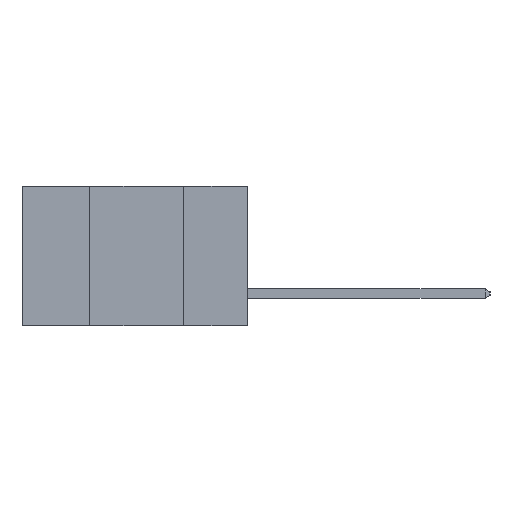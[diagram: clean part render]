
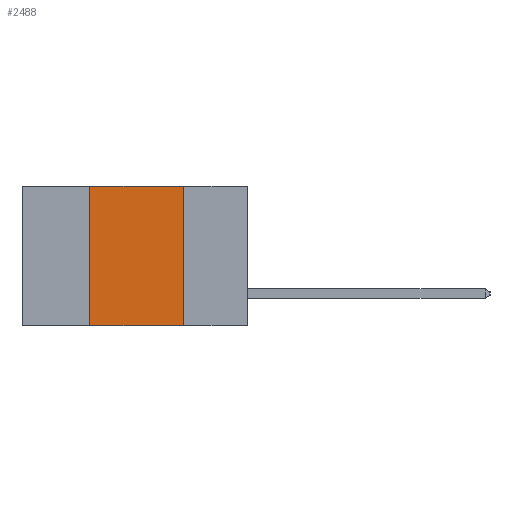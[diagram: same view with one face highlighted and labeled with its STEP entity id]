
A CAD part, left-side view. The second image highlights one B-rep face of the part: STEP entity #2488.
In plain terms, the highlighted planar face has unit normal (-1, 0, 0).
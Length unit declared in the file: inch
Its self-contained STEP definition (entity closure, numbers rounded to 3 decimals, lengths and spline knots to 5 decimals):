
#501 = VECTOR ( 'NONE', #7638, 39.37008 ) ;
#906 = VERTEX_POINT ( 'NONE', #5778 ) ;
#1119 = LINE ( 'NONE', #5964, #3027 ) ;
#1732 = CARTESIAN_POINT ( 'NONE',  ( 0., 0.6, 0. ) ) ;
#1875 = DIRECTION ( 'NONE',  ( 1., 0., 0. ) ) ;
#1886 = PLANE ( 'NONE',  #6725 ) ;
#2361 = CARTESIAN_POINT ( 'NONE',  ( 0., 0.42, -0.37 ) ) ;
#2488 = ADVANCED_FACE ( 'NONE', ( #5977 ), #1886, .F. ) ;
#2802 = VECTOR ( 'NONE', #7227, 39.37008 ) ;
#3027 = VECTOR ( 'NONE', #8045, 39.37008 ) ;
#3771 = CARTESIAN_POINT ( 'NONE',  ( 0., 0.42, 0. ) ) ;
#3807 = ORIENTED_EDGE ( 'NONE', *, *, #7808, .T. ) ;
#3818 = EDGE_CURVE ( 'NONE', #4007, #5707, #1119, .T. ) ;
#3910 = DIRECTION ( 'NONE',  ( 0., 0., -1. ) ) ;
#4007 = VERTEX_POINT ( 'NONE', #2361 ) ;
#4723 = VERTEX_POINT ( 'NONE', #6996 ) ;
#4745 = EDGE_LOOP ( 'NONE', ( #7411, #4828, #6081, #3807 ) ) ;
#4828 = ORIENTED_EDGE ( 'NONE', *, *, #9180, .F. ) ;
#5085 = VECTOR ( 'NONE', #6623, 39.37008 ) ;
#5707 = VERTEX_POINT ( 'NONE', #3771 ) ;
#5778 = CARTESIAN_POINT ( 'NONE',  ( 0., 0.17, 0. ) ) ;
#5935 = CARTESIAN_POINT ( 'NONE',  ( 0., 0.17, -0.37 ) ) ;
#5964 = CARTESIAN_POINT ( 'NONE',  ( 0., 0.42, -0.37 ) ) ;
#5977 = FACE_OUTER_BOUND ( 'NONE', #4745, .T. ) ;
#6081 = ORIENTED_EDGE ( 'NONE', *, *, #3818, .F. ) ;
#6526 = CARTESIAN_POINT ( 'NONE',  ( 0., 0.6, 0. ) ) ;
#6623 = DIRECTION ( 'NONE',  ( 0., 0., -1. ) ) ;
#6725 = AXIS2_PLACEMENT_3D ( 'NONE', #1732, #1875, #3910 ) ;
#6851 = LINE ( 'NONE', #6526, #2802 ) ;
#6951 = CARTESIAN_POINT ( 'NONE',  ( 0., 0.6, -0.37 ) ) ;
#6996 = CARTESIAN_POINT ( 'NONE',  ( 0., 0.17, -0.37 ) ) ;
#7227 = DIRECTION ( 'NONE',  ( 0., -1., 0. ) ) ;
#7411 = ORIENTED_EDGE ( 'NONE', *, *, #8133, .F. ) ;
#7638 = DIRECTION ( 'NONE',  ( 0., -1., 0. ) ) ;
#7808 = EDGE_CURVE ( 'NONE', #4007, #4723, #7828, .T. ) ;
#7828 = LINE ( 'NONE', #6951, #501 ) ;
#8045 = DIRECTION ( 'NONE',  ( 0., 0., 1. ) ) ;
#8133 = EDGE_CURVE ( 'NONE', #906, #4723, #8804, .T. ) ;
#8804 = LINE ( 'NONE', #5935, #5085 ) ;
#9180 = EDGE_CURVE ( 'NONE', #5707, #906, #6851, .T. ) ;
